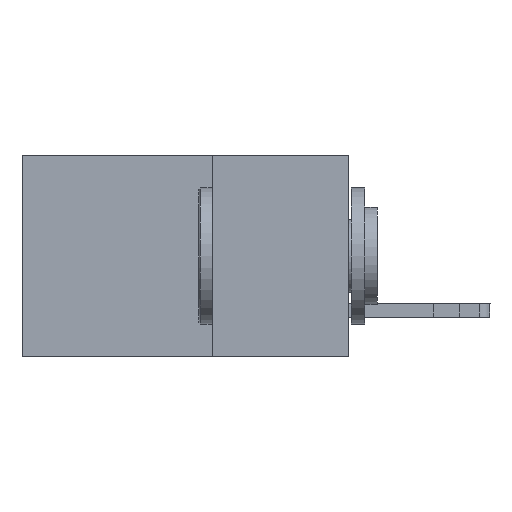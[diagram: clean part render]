
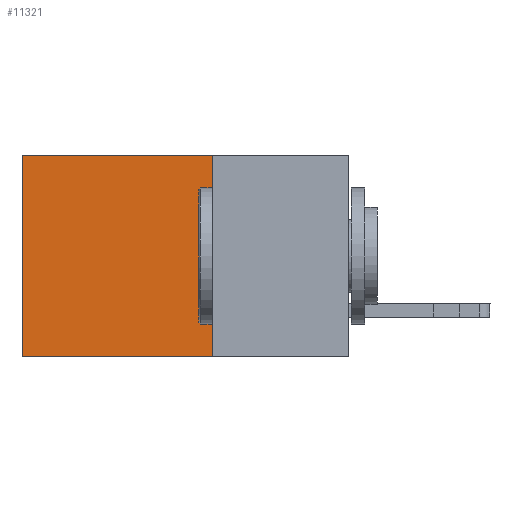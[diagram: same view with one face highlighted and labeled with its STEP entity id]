
A CAD part, left-side view. The second image highlights one B-rep face of the part: STEP entity #11321.
In plain terms, the highlighted planar face has unit normal (-1, 0, 0).
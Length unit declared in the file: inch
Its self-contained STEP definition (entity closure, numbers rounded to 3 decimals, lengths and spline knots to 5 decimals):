
#442 = ORIENTED_EDGE ( 'NONE', *, *, #2008, .T. ) ;
#784 = AXIS2_PLACEMENT_3D ( 'NONE', #2599, #3875, #12204 ) ;
#934 = LINE ( 'NONE', #2261, #13404 ) ;
#1461 = EDGE_CURVE ( 'NONE', #6310, #3899, #12129, .T. ) ;
#1508 = ORIENTED_EDGE ( 'NONE', *, *, #2348, .F. ) ;
#2008 = EDGE_CURVE ( 'NONE', #10671, #11579, #4322, .T. ) ;
#2261 = CARTESIAN_POINT ( 'NONE',  ( 0.2615, 0.25, 0. ) ) ;
#2348 = EDGE_CURVE ( 'NONE', #3899, #11579, #5824, .T. ) ;
#2516 = VECTOR ( 'NONE', #8935, 39.37008 ) ;
#2599 = CARTESIAN_POINT ( 'NONE',  ( 0.2615, 0.25, -0.37 ) ) ;
#2748 = CARTESIAN_POINT ( 'NONE',  ( 0.2615, 0.25, 0. ) ) ;
#3875 = DIRECTION ( 'NONE',  ( 1., 0., 0. ) ) ;
#3899 = VERTEX_POINT ( 'NONE', #4380 ) ;
#4322 = LINE ( 'NONE', #8309, #13390 ) ;
#4380 = CARTESIAN_POINT ( 'NONE',  ( 0.2615, 0.25, -0.37 ) ) ;
#4684 = ORIENTED_EDGE ( 'NONE', *, *, #6062, .T. ) ;
#4702 = EDGE_LOOP ( 'NONE', ( #442, #1508, #13755, #4684 ) ) ;
#4786 = DIRECTION ( 'NONE',  ( 0., 1., 0. ) ) ;
#5824 = LINE ( 'NONE', #13788, #2516 ) ;
#6062 = EDGE_CURVE ( 'NONE', #6310, #10671, #934, .T. ) ;
#6310 = VERTEX_POINT ( 'NONE', #2748 ) ;
#6748 = CARTESIAN_POINT ( 'NONE',  ( 0.2615, 0.25, -0.37 ) ) ;
#7729 = DIRECTION ( 'NONE',  ( 0., 0., -1. ) ) ;
#8157 = DIRECTION ( 'NONE',  ( 0., 0., -1. ) ) ;
#8309 = CARTESIAN_POINT ( 'NONE',  ( 0.2615, 0.6, -0.37 ) ) ;
#8709 = VECTOR ( 'NONE', #7729, 39.37008 ) ;
#8935 = DIRECTION ( 'NONE',  ( 0., 1., 0. ) ) ;
#9890 = PLANE ( 'NONE',  #784 ) ;
#10671 = VERTEX_POINT ( 'NONE', #11008 ) ;
#11008 = CARTESIAN_POINT ( 'NONE',  ( 0.2615, 0.6, 0. ) ) ;
#11321 = ADVANCED_FACE ( 'NONE', ( #13179 ), #9890, .F. ) ;
#11579 = VERTEX_POINT ( 'NONE', #12631 ) ;
#12129 = LINE ( 'NONE', #6748, #8709 ) ;
#12204 = DIRECTION ( 'NONE',  ( 0., 0., -1. ) ) ;
#12631 = CARTESIAN_POINT ( 'NONE',  ( 0.2615, 0.6, -0.37 ) ) ;
#13179 = FACE_OUTER_BOUND ( 'NONE', #4702, .T. ) ;
#13390 = VECTOR ( 'NONE', #8157, 39.37008 ) ;
#13404 = VECTOR ( 'NONE', #4786, 39.37008 ) ;
#13755 = ORIENTED_EDGE ( 'NONE', *, *, #1461, .F. ) ;
#13788 = CARTESIAN_POINT ( 'NONE',  ( 0.2615, 0.25, -0.37 ) ) ;
